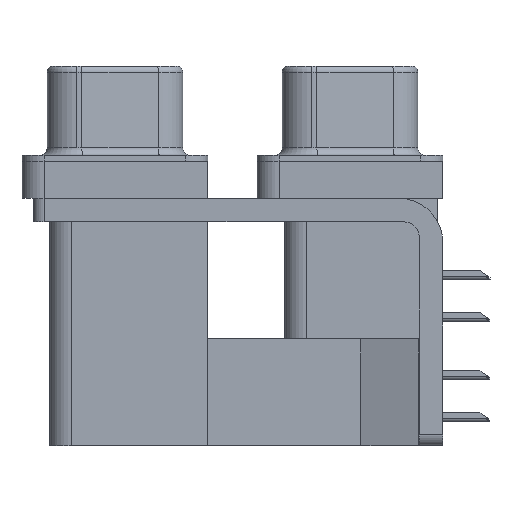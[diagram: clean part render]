
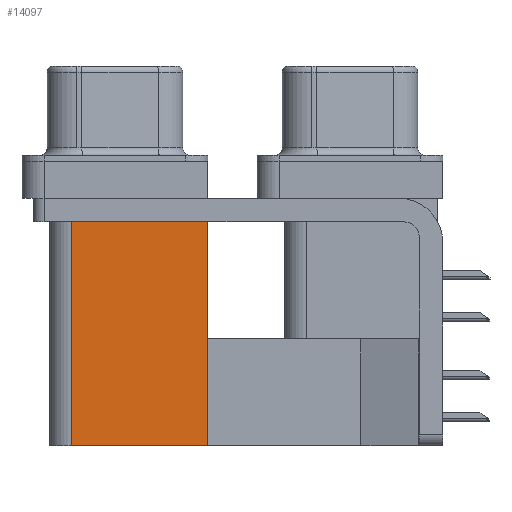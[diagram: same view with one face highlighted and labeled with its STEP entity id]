
A CAD part, left-side view. The second image highlights one B-rep face of the part: STEP entity #14097.
In plain terms, the highlighted planar face has unit normal (-1, 0, 0).
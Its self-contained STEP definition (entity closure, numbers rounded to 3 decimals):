
#155 = LINE ( 'NONE', #20053, #10684 ) ;
#1733 = CARTESIAN_POINT ( 'NONE',  ( 3.79, 9.6, -19.2 ) ) ;
#2238 = DIRECTION ( 'NONE',  ( 0., 0., 1. ) ) ;
#2503 = EDGE_CURVE ( 'NONE', #9388, #4454, #11971, .T. ) ;
#3873 = CARTESIAN_POINT ( 'NONE',  ( 3.79, 18.8, -2.5 ) ) ;
#3994 = CARTESIAN_POINT ( 'NONE',  ( 3.79, 9.6, -19.2 ) ) ;
#4136 = LINE ( 'NONE', #15970, #13660 ) ;
#4149 = CARTESIAN_POINT ( 'NONE',  ( 3.79, 9.6, -19.2 ) ) ;
#4301 = CARTESIAN_POINT ( 'NONE',  ( 3.79, 18.8, -19.2 ) ) ;
#4454 = VERTEX_POINT ( 'NONE', #3873 ) ;
#5004 = AXIS2_PLACEMENT_3D ( 'NONE', #4149, #8171, #14398 ) ;
#5171 = EDGE_CURVE ( 'NONE', #19197, #15081, #155, .T. ) ;
#5928 = VECTOR ( 'NONE', #12425, 1000. ) ;
#8088 = DIRECTION ( 'NONE',  ( 0., 0., 1. ) ) ;
#8171 = DIRECTION ( 'NONE',  ( 1., 0., 0. ) ) ;
#9388 = VERTEX_POINT ( 'NONE', #4301 ) ;
#10684 = VECTOR ( 'NONE', #2238, 1000. ) ;
#11971 = LINE ( 'NONE', #19924, #24826 ) ;
#12425 = DIRECTION ( 'NONE',  ( 0., 1., 0. ) ) ;
#13660 = VECTOR ( 'NONE', #23901, 1000. ) ;
#14097 = ADVANCED_FACE ( 'NONE', ( #20400 ), #18190, .F. ) ;
#14398 = DIRECTION ( 'NONE',  ( 0., 0., -1. ) ) ;
#15081 = VERTEX_POINT ( 'NONE', #16186 ) ;
#15858 = EDGE_CURVE ( 'NONE', #19197, #9388, #15959, .T. ) ;
#15959 = LINE ( 'NONE', #3994, #5928 ) ;
#15970 = CARTESIAN_POINT ( 'NONE',  ( 3.79, 9.6, -2.5 ) ) ;
#16186 = CARTESIAN_POINT ( 'NONE',  ( 3.79, 9.6, -2.5 ) ) ;
#16863 = ORIENTED_EDGE ( 'NONE', *, *, #24874, .T. ) ;
#18190 = PLANE ( 'NONE',  #5004 ) ;
#19197 = VERTEX_POINT ( 'NONE', #1733 ) ;
#19924 = CARTESIAN_POINT ( 'NONE',  ( 3.79, 18.8, -19.2 ) ) ;
#20053 = CARTESIAN_POINT ( 'NONE',  ( 3.79, 9.6, -19.2 ) ) ;
#20400 = FACE_OUTER_BOUND ( 'NONE', #20436, .T. ) ;
#20436 = EDGE_LOOP ( 'NONE', ( #16863, #21728, #23893, #22337 ) ) ;
#21728 = ORIENTED_EDGE ( 'NONE', *, *, #2503, .F. ) ;
#22337 = ORIENTED_EDGE ( 'NONE', *, *, #5171, .T. ) ;
#23893 = ORIENTED_EDGE ( 'NONE', *, *, #15858, .F. ) ;
#23901 = DIRECTION ( 'NONE',  ( 0., 1., 0. ) ) ;
#24826 = VECTOR ( 'NONE', #8088, 1000. ) ;
#24874 = EDGE_CURVE ( 'NONE', #15081, #4454, #4136, .T. ) ;
